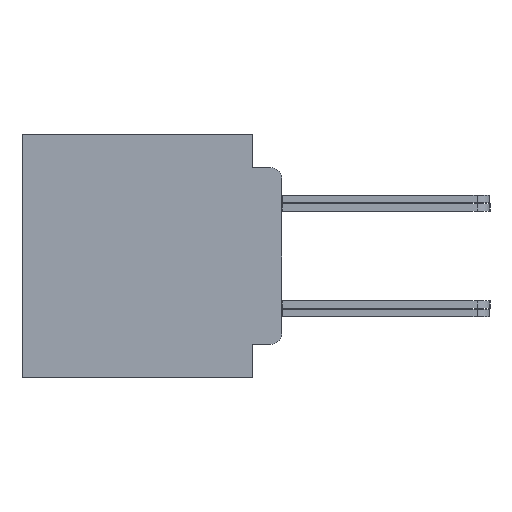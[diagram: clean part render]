
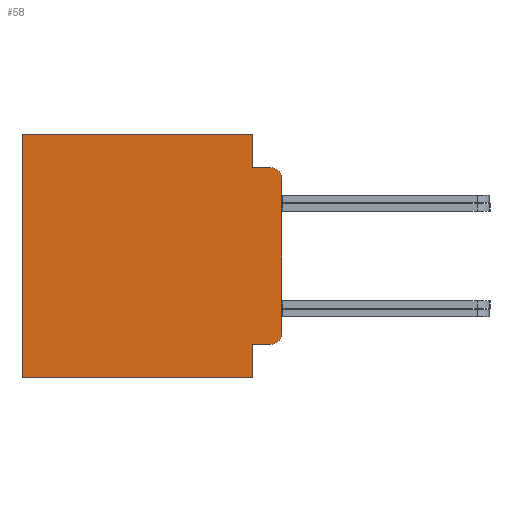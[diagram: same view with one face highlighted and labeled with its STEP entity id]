
A CAD part, left-side view. The second image highlights one B-rep face of the part: STEP entity #58.
In plain terms, the highlighted planar face has unit normal (-1, 0, 0).
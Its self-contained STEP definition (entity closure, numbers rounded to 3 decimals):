
#24 = CARTESIAN_POINT ( 'NONE',  ( -67.462, 11.684, -5.486 ) ) ;
#58 = ADVANCED_FACE ( 'NONE', ( #16852 ), #7572, .F. ) ;
#80 = LINE ( 'NONE', #3849, #24979 ) ;
#371 = DIRECTION ( 'NONE',  ( 0., 0., -1. ) ) ;
#1042 = VERTEX_POINT ( 'NONE', #24 ) ;
#1099 = DIRECTION ( 'NONE',  ( 1., 0., 0. ) ) ;
#1520 = EDGE_CURVE ( 'NONE', #9174, #27652, #11711, .T. ) ;
#1671 = DIRECTION ( 'NONE',  ( 0., 0., -1. ) ) ;
#2213 = EDGE_CURVE ( 'NONE', #24903, #21711, #7234, .T. ) ;
#2657 = ORIENTED_EDGE ( 'NONE', *, *, #21110, .F. ) ;
#2787 = VERTEX_POINT ( 'NONE', #26325 ) ;
#3298 = CARTESIAN_POINT ( 'NONE',  ( -67.462, 1.295, 5.486 ) ) ;
#3849 = CARTESIAN_POINT ( 'NONE',  ( -67.462, 11.684, -5.486 ) ) ;
#4436 = DIRECTION ( 'NONE',  ( 0., 0., -1. ) ) ;
#4735 = DIRECTION ( 'NONE',  ( -1., 0., 0. ) ) ;
#5086 = VERTEX_POINT ( 'NONE', #27492 ) ;
#5144 = CARTESIAN_POINT ( 'NONE',  ( -67.462, 1.295, 3.975 ) ) ;
#5914 = VECTOR ( 'NONE', #25914, 1000. ) ;
#6122 = CIRCLE ( 'NONE', #7438, 0.508 ) ;
#6300 = EDGE_CURVE ( 'NONE', #5086, #9174, #10312, .T. ) ;
#6684 = EDGE_CURVE ( 'NONE', #28239, #24903, #14728, .T. ) ;
#6809 = DIRECTION ( 'NONE',  ( 0., 0., -1. ) ) ;
#7234 = LINE ( 'NONE', #5144, #24297 ) ;
#7438 = AXIS2_PLACEMENT_3D ( 'NONE', #20330, #4735, #371 ) ;
#7572 = PLANE ( 'NONE',  #19418 ) ;
#7625 = LINE ( 'NONE', #26095, #5914 ) ;
#8633 = LINE ( 'NONE', #20006, #24680 ) ;
#8646 = AXIS2_PLACEMENT_3D ( 'NONE', #10839, #17476, #4436 ) ;
#9174 = VERTEX_POINT ( 'NONE', #26011 ) ;
#10312 = LINE ( 'NONE', #26623, #24649 ) ;
#10321 = VECTOR ( 'NONE', #13196, 1000. ) ;
#10839 = CARTESIAN_POINT ( 'NONE',  ( -67.462, 0.508, -3.467 ) ) ;
#10866 = VERTEX_POINT ( 'NONE', #24449 ) ;
#10937 = ORIENTED_EDGE ( 'NONE', *, *, #1520, .T. ) ;
#11560 = ORIENTED_EDGE ( 'NONE', *, *, #6684, .F. ) ;
#11711 = CIRCLE ( 'NONE', #8646, 0.508 ) ;
#11790 = EDGE_CURVE ( 'NONE', #28239, #12182, #7625, .T. ) ;
#11897 = ORIENTED_EDGE ( 'NONE', *, *, #11790, .T. ) ;
#12182 = VERTEX_POINT ( 'NONE', #27319 ) ;
#12259 = DIRECTION ( 'NONE',  ( 0., 1., 0. ) ) ;
#13196 = DIRECTION ( 'NONE',  ( 0., 0., -1. ) ) ;
#13880 = EDGE_CURVE ( 'NONE', #10866, #27652, #8633, .T. ) ;
#14230 = CARTESIAN_POINT ( 'NONE',  ( -67.462, 0.508, 3.975 ) ) ;
#14644 = CARTESIAN_POINT ( 'NONE',  ( -67.462, 0., -5.486 ) ) ;
#14728 = LINE ( 'NONE', #19169, #17786 ) ;
#14997 = DIRECTION ( 'NONE',  ( 0., 0., -1. ) ) ;
#15405 = ORIENTED_EDGE ( 'NONE', *, *, #2213, .F. ) ;
#15584 = ORIENTED_EDGE ( 'NONE', *, *, #6300, .T. ) ;
#15811 = DIRECTION ( 'NONE',  ( 0., -1., 0. ) ) ;
#16852 = FACE_OUTER_BOUND ( 'NONE', #21206, .T. ) ;
#16915 = LINE ( 'NONE', #14644, #17604 ) ;
#17100 = ORIENTED_EDGE ( 'NONE', *, *, #26321, .F. ) ;
#17476 = DIRECTION ( 'NONE',  ( -1., 0., 0. ) ) ;
#17604 = VECTOR ( 'NONE', #12259, 1000. ) ;
#17786 = VECTOR ( 'NONE', #21565, 1000. ) ;
#17876 = CARTESIAN_POINT ( 'NONE',  ( -67.462, 1.295, 0. ) ) ;
#18134 = CARTESIAN_POINT ( 'NONE',  ( -67.462, 0., -3.467 ) ) ;
#19169 = CARTESIAN_POINT ( 'NONE',  ( -67.462, 1.295, 0. ) ) ;
#19418 = AXIS2_PLACEMENT_3D ( 'NONE', #23622, #1099, #1671 ) ;
#19688 = ORIENTED_EDGE ( 'NONE', *, *, #13880, .F. ) ;
#20006 = CARTESIAN_POINT ( 'NONE',  ( -67.462, 0., -5.486 ) ) ;
#20330 = CARTESIAN_POINT ( 'NONE',  ( -67.462, 0.508, 3.467 ) ) ;
#20802 = ORIENTED_EDGE ( 'NONE', *, *, #27149, .T. ) ;
#21110 = EDGE_CURVE ( 'NONE', #2787, #1042, #16915, .T. ) ;
#21206 = EDGE_LOOP ( 'NONE', ( #15584, #10937, #19688, #25259, #15405, #11560, #11897, #20802, #2657, #17100 ) ) ;
#21565 = DIRECTION ( 'NONE',  ( 0., 0., -1. ) ) ;
#21711 = VERTEX_POINT ( 'NONE', #14230 ) ;
#22253 = DIRECTION ( 'NONE',  ( 0., -1., 0. ) ) ;
#23622 = CARTESIAN_POINT ( 'NONE',  ( -67.462, 0., -5.486 ) ) ;
#23978 = LINE ( 'NONE', #17876, #10321 ) ;
#24297 = VECTOR ( 'NONE', #22253, 1000. ) ;
#24449 = CARTESIAN_POINT ( 'NONE',  ( -67.462, 0., 3.467 ) ) ;
#24649 = VECTOR ( 'NONE', #15811, 1000. ) ;
#24680 = VECTOR ( 'NONE', #6809, 1000. ) ;
#24903 = VERTEX_POINT ( 'NONE', #26364 ) ;
#24979 = VECTOR ( 'NONE', #14997, 1000. ) ;
#25259 = ORIENTED_EDGE ( 'NONE', *, *, #28183, .T. ) ;
#25914 = DIRECTION ( 'NONE',  ( 0., 1., 0. ) ) ;
#26011 = CARTESIAN_POINT ( 'NONE',  ( -67.462, 0.508, -3.975 ) ) ;
#26095 = CARTESIAN_POINT ( 'NONE',  ( -67.462, 0., 5.486 ) ) ;
#26321 = EDGE_CURVE ( 'NONE', #5086, #2787, #23978, .T. ) ;
#26325 = CARTESIAN_POINT ( 'NONE',  ( -67.462, 1.295, -5.486 ) ) ;
#26364 = CARTESIAN_POINT ( 'NONE',  ( -67.462, 1.295, 3.975 ) ) ;
#26623 = CARTESIAN_POINT ( 'NONE',  ( -67.462, 1.295, -3.975 ) ) ;
#27149 = EDGE_CURVE ( 'NONE', #12182, #1042, #80, .T. ) ;
#27319 = CARTESIAN_POINT ( 'NONE',  ( -67.462, 11.684, 5.486 ) ) ;
#27492 = CARTESIAN_POINT ( 'NONE',  ( -67.462, 1.295, -3.975 ) ) ;
#27652 = VERTEX_POINT ( 'NONE', #18134 ) ;
#28183 = EDGE_CURVE ( 'NONE', #10866, #21711, #6122, .T. ) ;
#28239 = VERTEX_POINT ( 'NONE', #3298 ) ;
